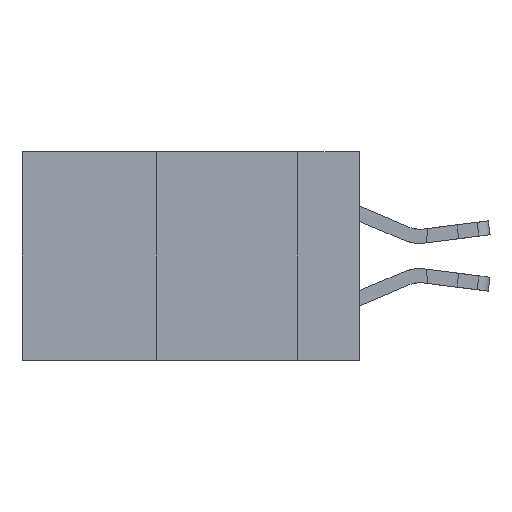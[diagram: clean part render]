
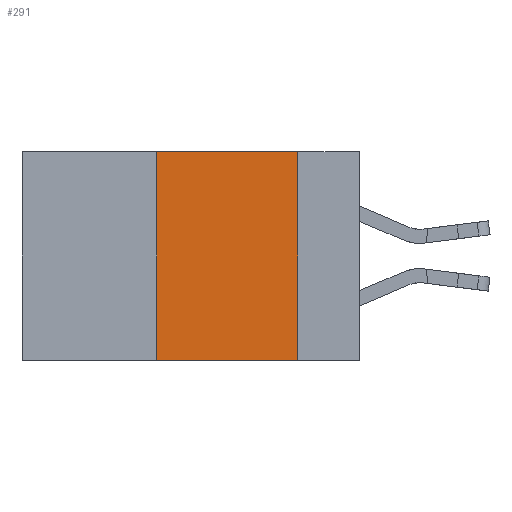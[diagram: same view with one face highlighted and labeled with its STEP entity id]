
A CAD part, left-side view. The second image highlights one B-rep face of the part: STEP entity #291.
In plain terms, the highlighted planar face has unit normal (-1, 0, 0).
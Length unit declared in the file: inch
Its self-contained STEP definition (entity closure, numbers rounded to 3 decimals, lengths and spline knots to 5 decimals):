
#291 = ADVANCED_FACE ( 'NONE', ( #21015 ), #16261, .F. ) ;
#376 = VECTOR ( 'NONE', #19474, 39.37008 ) ;
#2194 = ORIENTED_EDGE ( 'NONE', *, *, #6816, .F. ) ;
#2382 = LINE ( 'NONE', #19829, #20212 ) ;
#3076 = CARTESIAN_POINT ( 'NONE',  ( 0., 0.36, 0. ) ) ;
#3895 = LINE ( 'NONE', #12463, #12542 ) ;
#5004 = LINE ( 'NONE', #9075, #376 ) ;
#6816 = EDGE_CURVE ( 'NONE', #19525, #8051, #2382, .T. ) ;
#7674 = VERTEX_POINT ( 'NONE', #18826 ) ;
#7713 = CARTESIAN_POINT ( 'NONE',  ( 0., 0.11, 0. ) ) ;
#8051 = VERTEX_POINT ( 'NONE', #7713 ) ;
#8123 = VECTOR ( 'NONE', #18849, 39.37008 ) ;
#8460 = EDGE_CURVE ( 'NONE', #7674, #19525, #5004, .T. ) ;
#9075 = CARTESIAN_POINT ( 'NONE',  ( 0., 0.36, 0. ) ) ;
#9118 = CARTESIAN_POINT ( 'NONE',  ( 0., 0.11, -0.37 ) ) ;
#9660 = EDGE_CURVE ( 'NONE', #7674, #9714, #3895, .T. ) ;
#9692 = ORIENTED_EDGE ( 'NONE', *, *, #18369, .F. ) ;
#9714 = VERTEX_POINT ( 'NONE', #9118 ) ;
#10718 = DIRECTION ( 'NONE',  ( 0., -1., 0. ) ) ;
#11043 = AXIS2_PLACEMENT_3D ( 'NONE', #20509, #13356, #20889 ) ;
#12463 = CARTESIAN_POINT ( 'NONE',  ( 0., 0.6, -0.37 ) ) ;
#12542 = VECTOR ( 'NONE', #10718, 39.37008 ) ;
#13356 = DIRECTION ( 'NONE',  ( 1., 0., 0. ) ) ;
#14624 = DIRECTION ( 'NONE',  ( 0., -1., 0. ) ) ;
#15382 = CARTESIAN_POINT ( 'NONE',  ( 0., 0.11, 0. ) ) ;
#16261 = PLANE ( 'NONE',  #11043 ) ;
#18369 = EDGE_CURVE ( 'NONE', #8051, #9714, #21912, .T. ) ;
#18665 = EDGE_LOOP ( 'NONE', ( #9692, #2194, #19950, #19231 ) ) ;
#18826 = CARTESIAN_POINT ( 'NONE',  ( 0., 0.36, -0.37 ) ) ;
#18849 = DIRECTION ( 'NONE',  ( 0., 0., -1. ) ) ;
#19231 = ORIENTED_EDGE ( 'NONE', *, *, #9660, .T. ) ;
#19474 = DIRECTION ( 'NONE',  ( 0., 0., 1. ) ) ;
#19525 = VERTEX_POINT ( 'NONE', #3076 ) ;
#19829 = CARTESIAN_POINT ( 'NONE',  ( 0., 0.6, 0. ) ) ;
#19950 = ORIENTED_EDGE ( 'NONE', *, *, #8460, .F. ) ;
#20212 = VECTOR ( 'NONE', #14624, 39.37008 ) ;
#20509 = CARTESIAN_POINT ( 'NONE',  ( 0., 0.6, 0. ) ) ;
#20889 = DIRECTION ( 'NONE',  ( 0., 0., -1. ) ) ;
#21015 = FACE_OUTER_BOUND ( 'NONE', #18665, .T. ) ;
#21912 = LINE ( 'NONE', #15382, #8123 ) ;
